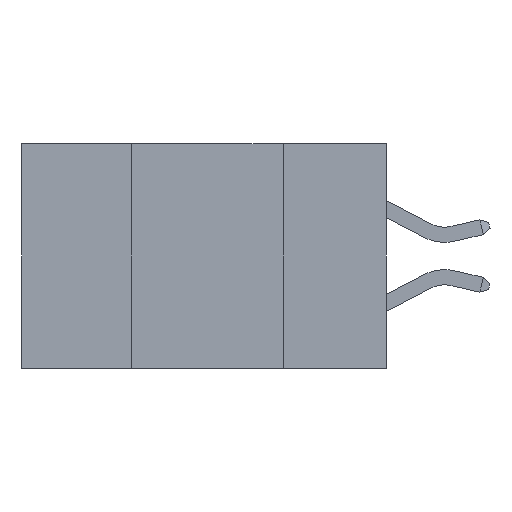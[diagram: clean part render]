
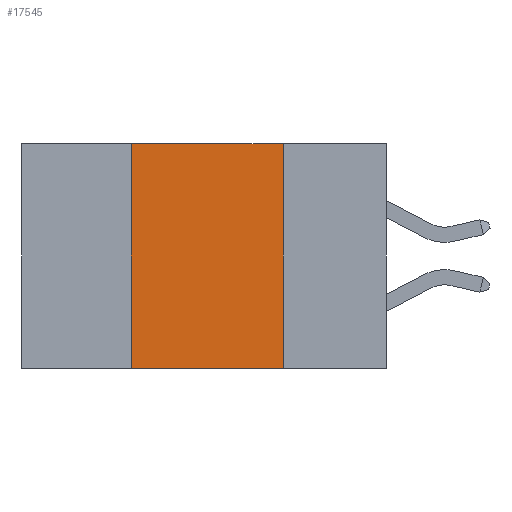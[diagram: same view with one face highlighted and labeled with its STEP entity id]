
A CAD part, left-side view. The second image highlights one B-rep face of the part: STEP entity #17545.
In plain terms, the highlighted planar face has unit normal (-1, 0, 0).
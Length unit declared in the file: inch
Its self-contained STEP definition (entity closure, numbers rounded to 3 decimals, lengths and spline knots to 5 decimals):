
#475 = VECTOR ( 'NONE', #15653, 39.37008 ) ;
#649 = DIRECTION ( 'NONE',  ( 0., 0., -1. ) ) ;
#1088 = LINE ( 'NONE', #23318, #475 ) ;
#1724 = VERTEX_POINT ( 'NONE', #19469 ) ;
#1859 = DIRECTION ( 'NONE',  ( 0., -1., 0. ) ) ;
#4152 = VECTOR ( 'NONE', #11778, 39.37008 ) ;
#5406 = EDGE_CURVE ( 'NONE', #19577, #1724, #14424, .T. ) ;
#5950 = CARTESIAN_POINT ( 'NONE',  ( 0., 0.42, 0. ) ) ;
#6861 = FACE_OUTER_BOUND ( 'NONE', #10285, .T. ) ;
#7142 = DIRECTION ( 'NONE',  ( 0., 0., -1. ) ) ;
#9104 = LINE ( 'NONE', #9723, #20558 ) ;
#9281 = EDGE_CURVE ( 'NONE', #20392, #22641, #9804, .T. ) ;
#9723 = CARTESIAN_POINT ( 'NONE',  ( 0., 0.6, -0.37 ) ) ;
#9804 = LINE ( 'NONE', #20607, #14320 ) ;
#10285 = EDGE_LOOP ( 'NONE', ( #18332, #23477, #14432, #19556 ) ) ;
#10384 = PLANE ( 'NONE',  #14394 ) ;
#11778 = DIRECTION ( 'NONE',  ( 0., 0., 1. ) ) ;
#12310 = DIRECTION ( 'NONE',  ( 1., 0., 0. ) ) ;
#14320 = VECTOR ( 'NONE', #7142, 39.37008 ) ;
#14394 = AXIS2_PLACEMENT_3D ( 'NONE', #23853, #12310, #649 ) ;
#14424 = LINE ( 'NONE', #5950, #4152 ) ;
#14432 = ORIENTED_EDGE ( 'NONE', *, *, #5406, .F. ) ;
#14447 = EDGE_CURVE ( 'NONE', #19577, #22641, #9104, .T. ) ;
#14824 = CARTESIAN_POINT ( 'NONE',  ( 0., 0.17, 0. ) ) ;
#15653 = DIRECTION ( 'NONE',  ( 0., -1., 0. ) ) ;
#16460 = CARTESIAN_POINT ( 'NONE',  ( 0., 0.42, -0.37 ) ) ;
#17545 = ADVANCED_FACE ( 'NONE', ( #6861 ), #10384, .F. ) ;
#18332 = ORIENTED_EDGE ( 'NONE', *, *, #9281, .F. ) ;
#18480 = CARTESIAN_POINT ( 'NONE',  ( 0., 0.17, -0.37 ) ) ;
#19469 = CARTESIAN_POINT ( 'NONE',  ( 0., 0.42, 0. ) ) ;
#19556 = ORIENTED_EDGE ( 'NONE', *, *, #14447, .T. ) ;
#19577 = VERTEX_POINT ( 'NONE', #16460 ) ;
#20392 = VERTEX_POINT ( 'NONE', #14824 ) ;
#20558 = VECTOR ( 'NONE', #1859, 39.37008 ) ;
#20607 = CARTESIAN_POINT ( 'NONE',  ( 0., 0.17, 0. ) ) ;
#20680 = EDGE_CURVE ( 'NONE', #1724, #20392, #1088, .T. ) ;
#22641 = VERTEX_POINT ( 'NONE', #18480 ) ;
#23318 = CARTESIAN_POINT ( 'NONE',  ( 0., 0.6, 0. ) ) ;
#23477 = ORIENTED_EDGE ( 'NONE', *, *, #20680, .F. ) ;
#23853 = CARTESIAN_POINT ( 'NONE',  ( 0., 0.6, 0. ) ) ;
